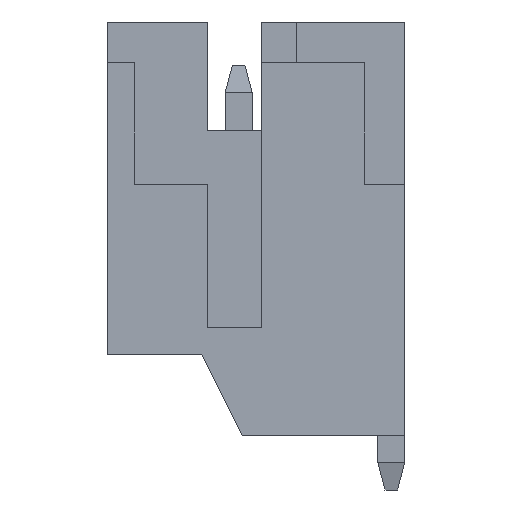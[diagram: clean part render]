
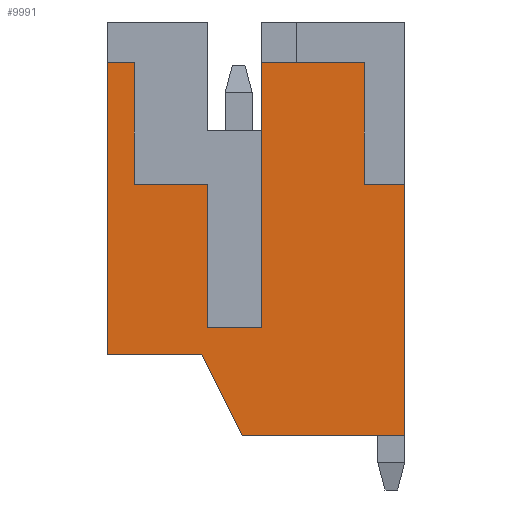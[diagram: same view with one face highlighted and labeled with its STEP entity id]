
A CAD part, left-side view. The second image highlights one B-rep face of the part: STEP entity #9991.
In plain terms, the highlighted planar face has unit normal (-1, 0, 0).
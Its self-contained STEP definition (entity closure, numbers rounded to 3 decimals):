
#150 = VERTEX_POINT ( 'NONE', #1409 ) ;
#260 = ORIENTED_EDGE ( 'NONE', *, *, #3591, .T. ) ;
#376 = CARTESIAN_POINT ( 'NONE',  ( -3., -3.07, -1.5 ) ) ;
#528 = DIRECTION ( 'NONE',  ( 0., -1., 0. ) ) ;
#529 = ORIENTED_EDGE ( 'NONE', *, *, #4466, .F. ) ;
#777 = CARTESIAN_POINT ( 'NONE',  ( -3., 0.68, 0. ) ) ;
#794 = LINE ( 'NONE', #1590, #9047 ) ;
#836 = DIRECTION ( 'NONE',  ( 0., 0., -1. ) ) ;
#902 = ORIENTED_EDGE ( 'NONE', *, *, #1393, .T. ) ;
#1033 = VECTOR ( 'NONE', #6986, 1000. ) ;
#1050 = VECTOR ( 'NONE', #7874, 1000. ) ;
#1090 = CARTESIAN_POINT ( 'NONE',  ( -3., -3.07, 3.15 ) ) ;
#1318 = PLANE ( 'NONE',  #5074 ) ;
#1393 = EDGE_CURVE ( 'NONE', #7401, #9410, #4982, .T. ) ;
#1409 = CARTESIAN_POINT ( 'NONE',  ( -3., 0.58, 3.15 ) ) ;
#1590 = CARTESIAN_POINT ( 'NONE',  ( -3., 2.43, 6.15 ) ) ;
#2059 = CARTESIAN_POINT ( 'NONE',  ( -3., -2.32, 3.15 ) ) ;
#2097 = VECTOR ( 'NONE', #9090, 1000. ) ;
#2106 = CARTESIAN_POINT ( 'NONE',  ( -3., -2.32, 3.15 ) ) ;
#2257 = ORIENTED_EDGE ( 'NONE', *, *, #9472, .T. ) ;
#2271 = VERTEX_POINT ( 'NONE', #9197 ) ;
#2318 = CARTESIAN_POINT ( 'NONE',  ( -3., -0.07, -1.5 ) ) ;
#2352 = LINE ( 'NONE', #376, #2097 ) ;
#2729 = DIRECTION ( 'NONE',  ( -1., 0., 0. ) ) ;
#2884 = DIRECTION ( 'NONE',  ( 0., 0., 1. ) ) ;
#2906 = CARTESIAN_POINT ( 'NONE',  ( -3., 2.43, 0. ) ) ;
#2997 = EDGE_CURVE ( 'NONE', #150, #6685, #5553, .T. ) ;
#3076 = CARTESIAN_POINT ( 'NONE',  ( -3., -0.42, 6.15 ) ) ;
#3163 = DIRECTION ( 'NONE',  ( 0., 0., 1. ) ) ;
#3276 = VERTEX_POINT ( 'NONE', #6593 ) ;
#3280 = CARTESIAN_POINT ( 'NONE',  ( -3., -2.32, 5.4 ) ) ;
#3324 = CARTESIAN_POINT ( 'NONE',  ( -3., -3.07, -1.5 ) ) ;
#3425 = VECTOR ( 'NONE', #8465, 1000. ) ;
#3575 = EDGE_CURVE ( 'NONE', #5242, #4133, #9689, .T. ) ;
#3591 = EDGE_CURVE ( 'NONE', #7112, #6642, #6672, .T. ) ;
#3675 = CARTESIAN_POINT ( 'NONE',  ( -3., -0.42, 3.15 ) ) ;
#3780 = ORIENTED_EDGE ( 'NONE', *, *, #8030, .T. ) ;
#4022 = ORIENTED_EDGE ( 'NONE', *, *, #3575, .T. ) ;
#4054 = EDGE_CURVE ( 'NONE', #3276, #7401, #794, .T. ) ;
#4133 = VERTEX_POINT ( 'NONE', #3280 ) ;
#4155 = ORIENTED_EDGE ( 'NONE', *, *, #8769, .T. ) ;
#4159 = VECTOR ( 'NONE', #5410, 1000. ) ;
#4380 = LINE ( 'NONE', #4570, #9775 ) ;
#4466 = EDGE_CURVE ( 'NONE', #6685, #7637, #4380, .T. ) ;
#4472 = CARTESIAN_POINT ( 'NONE',  ( -3., -2.32, 3.15 ) ) ;
#4500 = CARTESIAN_POINT ( 'NONE',  ( -3., -3.07, 5.4 ) ) ;
#4532 = ORIENTED_EDGE ( 'NONE', *, *, #8325, .T. ) ;
#4570 = CARTESIAN_POINT ( 'NONE',  ( -3., -0.42, 0.5 ) ) ;
#4982 = LINE ( 'NONE', #2906, #5115 ) ;
#5047 = CARTESIAN_POINT ( 'NONE',  ( -3., 0.58, 0.5 ) ) ;
#5074 = AXIS2_PLACEMENT_3D ( 'NONE', #6089, #2729, #7083 ) ;
#5086 = CARTESIAN_POINT ( 'NONE',  ( -3., 1.93, 3.15 ) ) ;
#5115 = VECTOR ( 'NONE', #7733, 1000. ) ;
#5143 = VECTOR ( 'NONE', #7166, 1000. ) ;
#5242 = VERTEX_POINT ( 'NONE', #2059 ) ;
#5410 = DIRECTION ( 'NONE',  ( 0., 1., 0. ) ) ;
#5414 = CARTESIAN_POINT ( 'NONE',  ( -3., -0.42, 5.4 ) ) ;
#5462 = EDGE_CURVE ( 'NONE', #5242, #6642, #9453, .T. ) ;
#5548 = VECTOR ( 'NONE', #3163, 1000. ) ;
#5553 = LINE ( 'NONE', #10031, #3425 ) ;
#5592 = CARTESIAN_POINT ( 'NONE',  ( -3., 1.93, 3.15 ) ) ;
#5743 = CARTESIAN_POINT ( 'NONE',  ( -3., -3.07, 5.4 ) ) ;
#5841 = ORIENTED_EDGE ( 'NONE', *, *, #9321, .T. ) ;
#6089 = CARTESIAN_POINT ( 'NONE',  ( -3., 0., 0. ) ) ;
#6282 = ORIENTED_EDGE ( 'NONE', *, *, #5462, .F. ) ;
#6465 = EDGE_LOOP ( 'NONE', ( #2257, #9122, #902, #4532, #9525, #260, #6282, #4022, #3780, #5841, #529, #7990, #7331, #4155 ) ) ;
#6573 = CARTESIAN_POINT ( 'NONE',  ( -3., -0.42, 0.5 ) ) ;
#6593 = CARTESIAN_POINT ( 'NONE',  ( -3., 2.43, 5.4 ) ) ;
#6642 = VERTEX_POINT ( 'NONE', #1090 ) ;
#6672 = LINE ( 'NONE', #10108, #8939 ) ;
#6685 = VERTEX_POINT ( 'NONE', #5047 ) ;
#6798 = LINE ( 'NONE', #4500, #4159 ) ;
#6964 = CARTESIAN_POINT ( 'NONE',  ( -3., -0.07, -1.5 ) ) ;
#6986 = DIRECTION ( 'NONE',  ( 0., -1., 0. ) ) ;
#7083 = DIRECTION ( 'NONE',  ( 0., -1., 0. ) ) ;
#7112 = VERTEX_POINT ( 'NONE', #3324 ) ;
#7166 = DIRECTION ( 'NONE',  ( 0., 0., -1. ) ) ;
#7201 = DIRECTION ( 'NONE',  ( 0., 1., 0. ) ) ;
#7282 = LINE ( 'NONE', #3076, #5143 ) ;
#7331 = ORIENTED_EDGE ( 'NONE', *, *, #9241, .F. ) ;
#7401 = VERTEX_POINT ( 'NONE', #7838 ) ;
#7523 = VECTOR ( 'NONE', #528, 1000. ) ;
#7637 = VERTEX_POINT ( 'NONE', #6573 ) ;
#7644 = DIRECTION ( 'NONE',  ( 0., 0., 1. ) ) ;
#7733 = DIRECTION ( 'NONE',  ( 0., -1., 0. ) ) ;
#7838 = CARTESIAN_POINT ( 'NONE',  ( -3., 2.43, 0. ) ) ;
#7872 = EDGE_CURVE ( 'NONE', #10284, #7112, #2352, .T. ) ;
#7874 = DIRECTION ( 'NONE',  ( 0., -0.447, -0.894 ) ) ;
#7990 = ORIENTED_EDGE ( 'NONE', *, *, #2997, .F. ) ;
#8030 = EDGE_CURVE ( 'NONE', #4133, #9172, #6798, .T. ) ;
#8149 = FACE_OUTER_BOUND ( 'NONE', #6465, .T. ) ;
#8167 = VECTOR ( 'NONE', #7201, 1000. ) ;
#8295 = LINE ( 'NONE', #3675, #1033 ) ;
#8305 = VECTOR ( 'NONE', #2884, 1000. ) ;
#8325 = EDGE_CURVE ( 'NONE', #9410, #10284, #9825, .T. ) ;
#8401 = VERTEX_POINT ( 'NONE', #5086 ) ;
#8465 = DIRECTION ( 'NONE',  ( 0., 0., -1. ) ) ;
#8769 = EDGE_CURVE ( 'NONE', #8401, #2271, #10074, .T. ) ;
#8939 = VECTOR ( 'NONE', #7644, 1000. ) ;
#9047 = VECTOR ( 'NONE', #836, 1000. ) ;
#9090 = DIRECTION ( 'NONE',  ( 0., -1., 0. ) ) ;
#9122 = ORIENTED_EDGE ( 'NONE', *, *, #4054, .T. ) ;
#9172 = VERTEX_POINT ( 'NONE', #5414 ) ;
#9197 = CARTESIAN_POINT ( 'NONE',  ( -3., 1.93, 5.4 ) ) ;
#9241 = EDGE_CURVE ( 'NONE', #8401, #150, #8295, .T. ) ;
#9321 = EDGE_CURVE ( 'NONE', #9172, #7637, #7282, .T. ) ;
#9373 = DIRECTION ( 'NONE',  ( 0., -1., 0. ) ) ;
#9410 = VERTEX_POINT ( 'NONE', #777 ) ;
#9453 = LINE ( 'NONE', #4472, #7523 ) ;
#9472 = EDGE_CURVE ( 'NONE', #2271, #3276, #9792, .T. ) ;
#9525 = ORIENTED_EDGE ( 'NONE', *, *, #7872, .T. ) ;
#9689 = LINE ( 'NONE', #2106, #8305 ) ;
#9775 = VECTOR ( 'NONE', #9373, 1000. ) ;
#9792 = LINE ( 'NONE', #5743, #8167 ) ;
#9825 = LINE ( 'NONE', #2318, #1050 ) ;
#9991 = ADVANCED_FACE ( 'NONE', ( #8149 ), #1318, .T. ) ;
#10031 = CARTESIAN_POINT ( 'NONE',  ( -3., 0.58, 3.15 ) ) ;
#10074 = LINE ( 'NONE', #5592, #5548 ) ;
#10108 = CARTESIAN_POINT ( 'NONE',  ( -3., -3.07, 6.15 ) ) ;
#10284 = VERTEX_POINT ( 'NONE', #6964 ) ;
